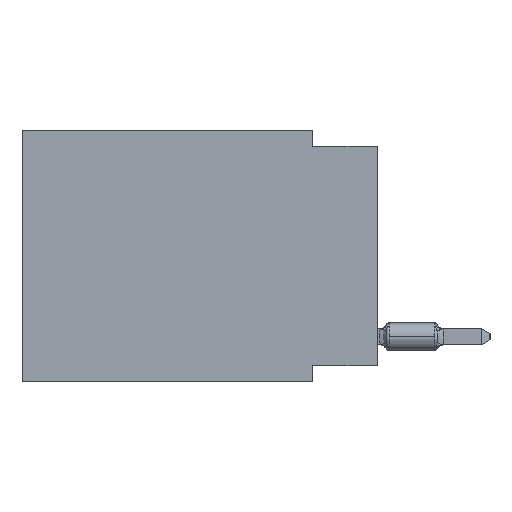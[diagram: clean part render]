
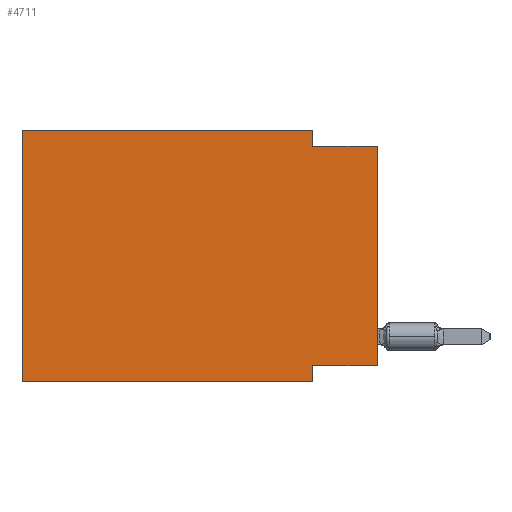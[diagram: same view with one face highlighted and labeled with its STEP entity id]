
A CAD part, left-side view. The second image highlights one B-rep face of the part: STEP entity #4711.
In plain terms, the highlighted planar face has unit normal (-1, 0, 0).
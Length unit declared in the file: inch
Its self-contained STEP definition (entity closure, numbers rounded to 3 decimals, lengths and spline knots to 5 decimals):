
#510 = CARTESIAN_POINT ( 'NONE',  ( 0., 0.55, 0. ) ) ;
#1499 = ORIENTED_EDGE ( 'NONE', *, *, #11607, .T. ) ;
#1579 = DIRECTION ( 'NONE',  ( 0., 0., -1. ) ) ;
#1750 = VERTEX_POINT ( 'NONE', #18488 ) ;
#3974 = VERTEX_POINT ( 'NONE', #40245 ) ;
#4711 = ADVANCED_FACE ( 'NONE', ( #39804 ), #33524, .F. ) ;
#5096 = LINE ( 'NONE', #41134, #21435 ) ;
#5167 = VERTEX_POINT ( 'NONE', #19777 ) ;
#5443 = ORIENTED_EDGE ( 'NONE', *, *, #32391, .F. ) ;
#5472 = LINE ( 'NONE', #22819, #37537 ) ;
#7297 = VERTEX_POINT ( 'NONE', #33375 ) ;
#8576 = LINE ( 'NONE', #28552, #21160 ) ;
#10461 = LINE ( 'NONE', #24129, #37886 ) ;
#11607 = EDGE_CURVE ( 'NONE', #7297, #5167, #23802, .T. ) ;
#14095 = EDGE_CURVE ( 'NONE', #34681, #1750, #10461, .T. ) ;
#14167 = DIRECTION ( 'NONE',  ( 0., 0., -1. ) ) ;
#15068 = DIRECTION ( 'NONE',  ( 0., -1., 0. ) ) ;
#15396 = VECTOR ( 'NONE', #40022, 39.37008 ) ;
#15765 = ORIENTED_EDGE ( 'NONE', *, *, #14095, .F. ) ;
#17136 = EDGE_CURVE ( 'NONE', #1750, #25231, #5096, .T. ) ;
#17695 = ORIENTED_EDGE ( 'NONE', *, *, #36734, .F. ) ;
#18283 = VECTOR ( 'NONE', #30982, 39.37008 ) ;
#18345 = VERTEX_POINT ( 'NONE', #30350 ) ;
#18488 = CARTESIAN_POINT ( 'NONE',  ( 0., 0.1, -0.025 ) ) ;
#19777 = CARTESIAN_POINT ( 'NONE',  ( 0., 0.1, -0.39 ) ) ;
#19838 = LINE ( 'NONE', #42860, #15396 ) ;
#20895 = EDGE_CURVE ( 'NONE', #7297, #3974, #30045, .T. ) ;
#21160 = VECTOR ( 'NONE', #38534, 39.37008 ) ;
#21247 = EDGE_CURVE ( 'NONE', #18345, #25231, #5472, .T. ) ;
#21435 = VECTOR ( 'NONE', #15068, 39.37008 ) ;
#22819 = CARTESIAN_POINT ( 'NONE',  ( 0., 0., 0. ) ) ;
#22869 = CARTESIAN_POINT ( 'NONE',  ( 0., 0.55, 0. ) ) ;
#23802 = LINE ( 'NONE', #24019, #18283 ) ;
#23941 = DIRECTION ( 'NONE',  ( 0., 0., 1. ) ) ;
#24019 = CARTESIAN_POINT ( 'NONE',  ( 0., 0.55, -0.39 ) ) ;
#24022 = EDGE_LOOP ( 'NONE', ( #37555, #38586, #15765, #17695, #27795, #1499, #5443, #32088 ) ) ;
#24129 = CARTESIAN_POINT ( 'NONE',  ( 0., 0.1, 0. ) ) ;
#25231 = VERTEX_POINT ( 'NONE', #34726 ) ;
#25776 = CARTESIAN_POINT ( 'NONE',  ( 0., 0.1, 0. ) ) ;
#26033 = AXIS2_PLACEMENT_3D ( 'NONE', #22869, #39594, #36127 ) ;
#27643 = CARTESIAN_POINT ( 'NONE',  ( 0., 0.1, -0.39 ) ) ;
#27795 = ORIENTED_EDGE ( 'NONE', *, *, #20895, .F. ) ;
#28552 = CARTESIAN_POINT ( 'NONE',  ( 0., 0.55, 0. ) ) ;
#30045 = LINE ( 'NONE', #510, #38181 ) ;
#30350 = CARTESIAN_POINT ( 'NONE',  ( 0., 0., -0.365 ) ) ;
#30982 = DIRECTION ( 'NONE',  ( 0., -1., 0. ) ) ;
#31844 = VERTEX_POINT ( 'NONE', #33354 ) ;
#32088 = ORIENTED_EDGE ( 'NONE', *, *, #33475, .F. ) ;
#32391 = EDGE_CURVE ( 'NONE', #31844, #5167, #34590, .T. ) ;
#32409 = DIRECTION ( 'NONE',  ( 0., 0., 1. ) ) ;
#33354 = CARTESIAN_POINT ( 'NONE',  ( 0., 0.1, -0.365 ) ) ;
#33375 = CARTESIAN_POINT ( 'NONE',  ( 0., 0.55, -0.39 ) ) ;
#33475 = EDGE_CURVE ( 'NONE', #18345, #31844, #19838, .T. ) ;
#33524 = PLANE ( 'NONE',  #26033 ) ;
#34590 = LINE ( 'NONE', #27643, #42432 ) ;
#34681 = VERTEX_POINT ( 'NONE', #25776 ) ;
#34726 = CARTESIAN_POINT ( 'NONE',  ( 0., 0., -0.025 ) ) ;
#36127 = DIRECTION ( 'NONE',  ( 0., 0., -1. ) ) ;
#36734 = EDGE_CURVE ( 'NONE', #3974, #34681, #8576, .T. ) ;
#37537 = VECTOR ( 'NONE', #32409, 39.37008 ) ;
#37555 = ORIENTED_EDGE ( 'NONE', *, *, #21247, .T. ) ;
#37886 = VECTOR ( 'NONE', #14167, 39.37008 ) ;
#38181 = VECTOR ( 'NONE', #23941, 39.37008 ) ;
#38534 = DIRECTION ( 'NONE',  ( 0., -1., 0. ) ) ;
#38586 = ORIENTED_EDGE ( 'NONE', *, *, #17136, .F. ) ;
#39594 = DIRECTION ( 'NONE',  ( 1., 0., 0. ) ) ;
#39804 = FACE_OUTER_BOUND ( 'NONE', #24022, .T. ) ;
#40022 = DIRECTION ( 'NONE',  ( 0., 1., 0. ) ) ;
#40245 = CARTESIAN_POINT ( 'NONE',  ( 0., 0.55, 0. ) ) ;
#41134 = CARTESIAN_POINT ( 'NONE',  ( 0., 0., -0.025 ) ) ;
#42432 = VECTOR ( 'NONE', #1579, 39.37008 ) ;
#42860 = CARTESIAN_POINT ( 'NONE',  ( 0., 0., -0.365 ) ) ;
